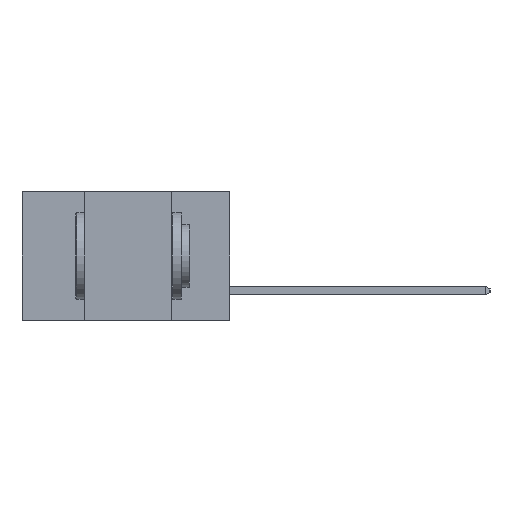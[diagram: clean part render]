
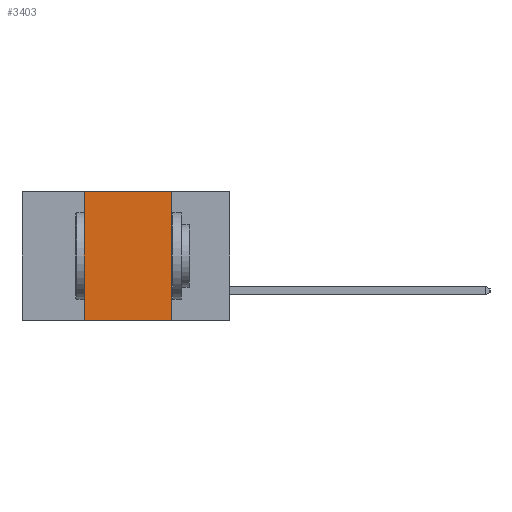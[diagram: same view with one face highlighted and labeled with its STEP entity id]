
A CAD part, left-side view. The second image highlights one B-rep face of the part: STEP entity #3403.
In plain terms, the highlighted planar face has unit normal (-1, 0, 0).
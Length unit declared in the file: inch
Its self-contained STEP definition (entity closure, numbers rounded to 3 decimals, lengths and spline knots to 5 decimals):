
#1651 = LINE ( 'NONE', #7689, #22043 ) ;
#2214 = LINE ( 'NONE', #9699, #21949 ) ;
#2603 = CARTESIAN_POINT ( 'NONE',  ( 0., 0.17, 0. ) ) ;
#2875 = VERTEX_POINT ( 'NONE', #20241 ) ;
#3037 = VECTOR ( 'NONE', #15632, 39.37008 ) ;
#3159 = ORIENTED_EDGE ( 'NONE', *, *, #9904, .T. ) ;
#3298 = EDGE_CURVE ( 'NONE', #10226, #11217, #8222, .T. ) ;
#3403 = ADVANCED_FACE ( 'NONE', ( #21361 ), #12547, .F. ) ;
#7281 = CARTESIAN_POINT ( 'NONE',  ( 0., 0.42, -0.37 ) ) ;
#7689 = CARTESIAN_POINT ( 'NONE',  ( 0., 0.6, 0. ) ) ;
#8082 = AXIS2_PLACEMENT_3D ( 'NONE', #13243, #12514, #12482 ) ;
#8222 = LINE ( 'NONE', #17168, #18019 ) ;
#9672 = DIRECTION ( 'NONE',  ( 0., -1., 0. ) ) ;
#9699 = CARTESIAN_POINT ( 'NONE',  ( 0., 0.42, -0.37 ) ) ;
#9904 = EDGE_CURVE ( 'NONE', #11874, #11217, #19415, .T. ) ;
#10226 = VERTEX_POINT ( 'NONE', #2603 ) ;
#11217 = VERTEX_POINT ( 'NONE', #18634 ) ;
#11819 = EDGE_LOOP ( 'NONE', ( #17702, #22819, #23420, #3159 ) ) ;
#11874 = VERTEX_POINT ( 'NONE', #7281 ) ;
#12482 = DIRECTION ( 'NONE',  ( 0., 0., -1. ) ) ;
#12514 = DIRECTION ( 'NONE',  ( 1., 0., 0. ) ) ;
#12547 = PLANE ( 'NONE',  #8082 ) ;
#13243 = CARTESIAN_POINT ( 'NONE',  ( 0., 0.6, 0. ) ) ;
#14087 = CARTESIAN_POINT ( 'NONE',  ( 0., 0.6, -0.37 ) ) ;
#15632 = DIRECTION ( 'NONE',  ( 0., -1., 0. ) ) ;
#17138 = DIRECTION ( 'NONE',  ( 0., 0., -1. ) ) ;
#17168 = CARTESIAN_POINT ( 'NONE',  ( 0., 0.17, -0.37 ) ) ;
#17702 = ORIENTED_EDGE ( 'NONE', *, *, #3298, .F. ) ;
#18019 = VECTOR ( 'NONE', #17138, 39.37008 ) ;
#18634 = CARTESIAN_POINT ( 'NONE',  ( 0., 0.17, -0.37 ) ) ;
#19415 = LINE ( 'NONE', #14087, #3037 ) ;
#20241 = CARTESIAN_POINT ( 'NONE',  ( 0., 0.42, 0. ) ) ;
#21302 = EDGE_CURVE ( 'NONE', #2875, #10226, #1651, .T. ) ;
#21361 = FACE_OUTER_BOUND ( 'NONE', #11819, .T. ) ;
#21402 = DIRECTION ( 'NONE',  ( 0., 0., 1. ) ) ;
#21949 = VECTOR ( 'NONE', #21402, 39.37008 ) ;
#22043 = VECTOR ( 'NONE', #9672, 39.37008 ) ;
#22819 = ORIENTED_EDGE ( 'NONE', *, *, #21302, .F. ) ;
#23420 = ORIENTED_EDGE ( 'NONE', *, *, #23547, .F. ) ;
#23547 = EDGE_CURVE ( 'NONE', #11874, #2875, #2214, .T. ) ;
